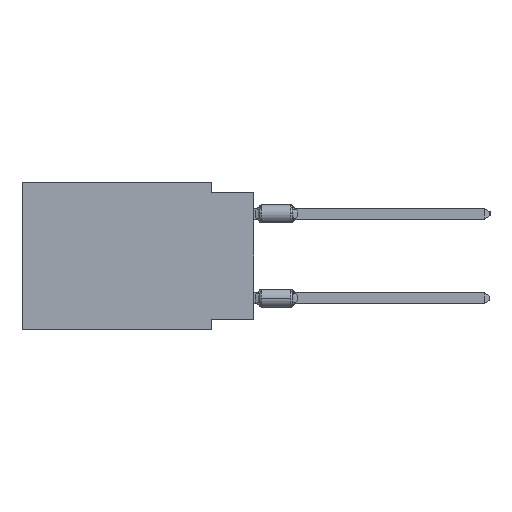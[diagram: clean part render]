
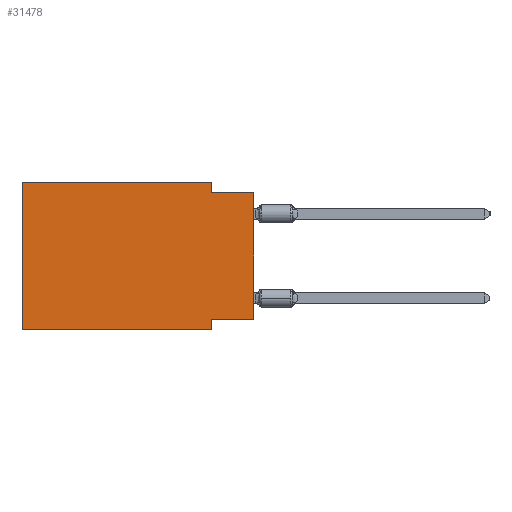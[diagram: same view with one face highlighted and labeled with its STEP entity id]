
A CAD part, left-side view. The second image highlights one B-rep face of the part: STEP entity #31478.
In plain terms, the highlighted planar face has unit normal (-1, 0, 0).
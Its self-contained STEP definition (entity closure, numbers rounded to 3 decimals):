
#316 = DIRECTION ( 'NONE',  ( 0., 0., 1. ) ) ;
#1808 = CARTESIAN_POINT ( 'NONE',  ( 0., 2.54, -8.255 ) ) ;
#2058 = PLANE ( 'NONE',  #44762 ) ;
#2912 = DIRECTION ( 'NONE',  ( 0., 0., -1. ) ) ;
#3767 = CARTESIAN_POINT ( 'NONE',  ( 0., 13.97, -8.89 ) ) ;
#5333 = ORIENTED_EDGE ( 'NONE', *, *, #6893, .F. ) ;
#5987 = VERTEX_POINT ( 'NONE', #3767 ) ;
#6893 = EDGE_CURVE ( 'NONE', #38992, #21290, #14998, .T. ) ;
#7155 = VECTOR ( 'NONE', #316, 1000. ) ;
#7379 = VECTOR ( 'NONE', #49600, 1000. ) ;
#7635 = CARTESIAN_POINT ( 'NONE',  ( 0., 2.54, 0. ) ) ;
#8241 = CARTESIAN_POINT ( 'NONE',  ( 0., 13.97, 0. ) ) ;
#11419 = DIRECTION ( 'NONE',  ( 0., -1., 0. ) ) ;
#11714 = EDGE_CURVE ( 'NONE', #35898, #38992, #30613, .T. ) ;
#11893 = DIRECTION ( 'NONE',  ( 0., -1., 0. ) ) ;
#12413 = CARTESIAN_POINT ( 'NONE',  ( 0., 0., -0.635 ) ) ;
#12432 = VECTOR ( 'NONE', #11893, 1000. ) ;
#12722 = ORIENTED_EDGE ( 'NONE', *, *, #47840, .F. ) ;
#13650 = CARTESIAN_POINT ( 'NONE',  ( 0., 13.97, 0. ) ) ;
#13924 = DIRECTION ( 'NONE',  ( 1., 0., 0. ) ) ;
#14322 = CARTESIAN_POINT ( 'NONE',  ( 0., 13.97, -8.89 ) ) ;
#14998 = LINE ( 'NONE', #31065, #48399 ) ;
#15047 = LINE ( 'NONE', #31115, #25259 ) ;
#16148 = LINE ( 'NONE', #8241, #7155 ) ;
#16966 = VERTEX_POINT ( 'NONE', #1808 ) ;
#18300 = LINE ( 'NONE', #14322, #28811 ) ;
#21290 = VERTEX_POINT ( 'NONE', #29266 ) ;
#22217 = LINE ( 'NONE', #12413, #12432 ) ;
#23483 = LINE ( 'NONE', #46417, #40603 ) ;
#25255 = ORIENTED_EDGE ( 'NONE', *, *, #33709, .T. ) ;
#25259 = VECTOR ( 'NONE', #37966, 1000. ) ;
#26536 = EDGE_CURVE ( 'NONE', #42712, #16966, #15047, .T. ) ;
#26757 = ORIENTED_EDGE ( 'NONE', *, *, #51248, .F. ) ;
#27474 = ORIENTED_EDGE ( 'NONE', *, *, #11714, .F. ) ;
#27873 = ORIENTED_EDGE ( 'NONE', *, *, #41578, .F. ) ;
#27959 = DIRECTION ( 'NONE',  ( 0., 0., 1. ) ) ;
#28811 = VECTOR ( 'NONE', #11419, 1000. ) ;
#29266 = CARTESIAN_POINT ( 'NONE',  ( 0., 2.54, -0.635 ) ) ;
#29358 = CARTESIAN_POINT ( 'NONE',  ( 0., 0., -8.255 ) ) ;
#29733 = ORIENTED_EDGE ( 'NONE', *, *, #26536, .F. ) ;
#29911 = CARTESIAN_POINT ( 'NONE',  ( 0., 0., -0.635 ) ) ;
#30613 = LINE ( 'NONE', #50647, #7379 ) ;
#31065 = CARTESIAN_POINT ( 'NONE',  ( 0., 2.54, 0. ) ) ;
#31115 = CARTESIAN_POINT ( 'NONE',  ( 0., 0., -8.255 ) ) ;
#31387 = LINE ( 'NONE', #35598, #50849 ) ;
#31478 = ADVANCED_FACE ( 'NONE', ( #37640 ), #2058, .F. ) ;
#32057 = CARTESIAN_POINT ( 'NONE',  ( 0., 13.97, 0. ) ) ;
#32388 = VERTEX_POINT ( 'NONE', #50969 ) ;
#32439 = EDGE_CURVE ( 'NONE', #5987, #32388, #18300, .T. ) ;
#33709 = EDGE_CURVE ( 'NONE', #42712, #47218, #31387, .T. ) ;
#33851 = ORIENTED_EDGE ( 'NONE', *, *, #32439, .T. ) ;
#35598 = CARTESIAN_POINT ( 'NONE',  ( 0., 0., 0. ) ) ;
#35898 = VERTEX_POINT ( 'NONE', #32057 ) ;
#37640 = FACE_OUTER_BOUND ( 'NONE', #49289, .T. ) ;
#37966 = DIRECTION ( 'NONE',  ( 0., 1., 0. ) ) ;
#38425 = DIRECTION ( 'NONE',  ( 0., 0., -1. ) ) ;
#38992 = VERTEX_POINT ( 'NONE', #7635 ) ;
#40603 = VECTOR ( 'NONE', #2912, 1000. ) ;
#41578 = EDGE_CURVE ( 'NONE', #16966, #32388, #23483, .T. ) ;
#42712 = VERTEX_POINT ( 'NONE', #29358 ) ;
#44762 = AXIS2_PLACEMENT_3D ( 'NONE', #13650, #13924, #38425 ) ;
#46417 = CARTESIAN_POINT ( 'NONE',  ( 0., 2.54, -8.89 ) ) ;
#47140 = DIRECTION ( 'NONE',  ( 0., 0., -1. ) ) ;
#47218 = VERTEX_POINT ( 'NONE', #29911 ) ;
#47840 = EDGE_CURVE ( 'NONE', #21290, #47218, #22217, .T. ) ;
#48399 = VECTOR ( 'NONE', #47140, 1000. ) ;
#49289 = EDGE_LOOP ( 'NONE', ( #25255, #12722, #5333, #27474, #26757, #33851, #27873, #29733 ) ) ;
#49600 = DIRECTION ( 'NONE',  ( 0., -1., 0. ) ) ;
#50647 = CARTESIAN_POINT ( 'NONE',  ( 0., 13.97, 0. ) ) ;
#50849 = VECTOR ( 'NONE', #27959, 1000. ) ;
#50969 = CARTESIAN_POINT ( 'NONE',  ( 0., 2.54, -8.89 ) ) ;
#51248 = EDGE_CURVE ( 'NONE', #5987, #35898, #16148, .T. ) ;
